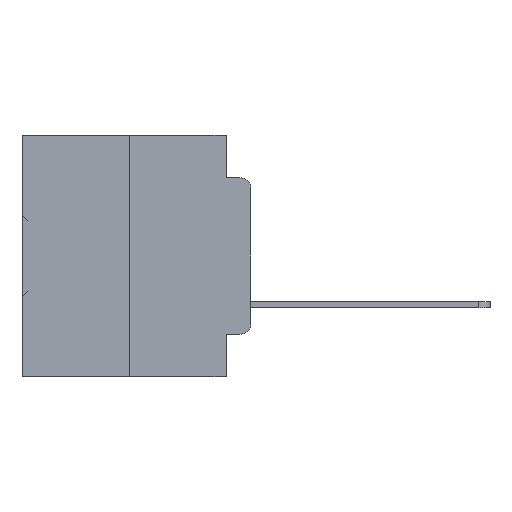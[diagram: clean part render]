
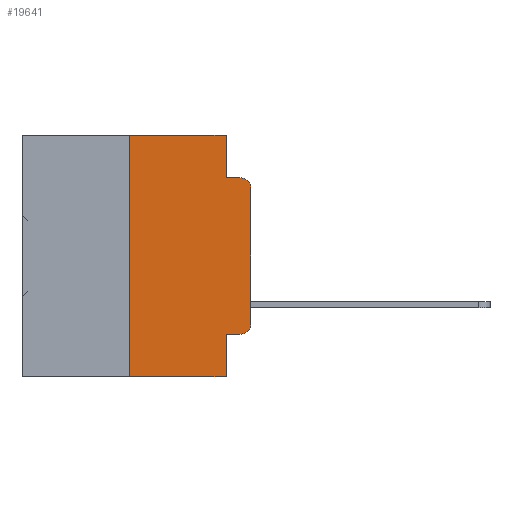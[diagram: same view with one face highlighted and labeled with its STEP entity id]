
A CAD part, left-side view. The second image highlights one B-rep face of the part: STEP entity #19641.
In plain terms, the highlighted planar face has unit normal (-1, 0, 0).
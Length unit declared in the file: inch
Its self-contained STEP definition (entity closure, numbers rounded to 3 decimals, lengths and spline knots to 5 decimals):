
#29 = CARTESIAN_POINT ( 'NONE',  ( 0., 0.25, 0. ) ) ;
#360 = DIRECTION ( 'NONE',  ( 0., -1., 0. ) ) ;
#1516 = VERTEX_POINT ( 'NONE', #3361 ) ;
#1761 = CIRCLE ( 'NONE', #10310, 0.02 ) ;
#1871 = PLANE ( 'NONE',  #21102 ) ;
#1958 = DIRECTION ( 'NONE',  ( 0., -1., 0. ) ) ;
#2050 = DIRECTION ( 'NONE',  ( 0., 0., -1. ) ) ;
#2464 = CARTESIAN_POINT ( 'NONE',  ( 0., 0.25, -0.5 ) ) ;
#2479 = CARTESIAN_POINT ( 'NONE',  ( 0., 0.051, 0. ) ) ;
#3361 = CARTESIAN_POINT ( 'NONE',  ( 0., 0.02, -0.4115 ) ) ;
#4525 = LINE ( 'NONE', #7889, #23903 ) ;
#4834 = DIRECTION ( 'NONE',  ( 1., 0., 0. ) ) ;
#5090 = DIRECTION ( 'NONE',  ( 0., 0., -1. ) ) ;
#5149 = CARTESIAN_POINT ( 'NONE',  ( 0., 0.02, -0.1085 ) ) ;
#5517 = EDGE_CURVE ( 'NONE', #33717, #28321, #29204, .T. ) ;
#5918 = ORIENTED_EDGE ( 'NONE', *, *, #34661, .F. ) ;
#6010 = CARTESIAN_POINT ( 'NONE',  ( 0., 0.25, 0. ) ) ;
#7038 = CARTESIAN_POINT ( 'NONE',  ( 0., 0., -0.1085 ) ) ;
#7889 = CARTESIAN_POINT ( 'NONE',  ( 0., 0.473, -0.5 ) ) ;
#9245 = ORIENTED_EDGE ( 'NONE', *, *, #11551, .T. ) ;
#9470 = DIRECTION ( 'NONE',  ( 0., 0., 1. ) ) ;
#10193 = VECTOR ( 'NONE', #360, 39.37008 ) ;
#10310 = AXIS2_PLACEMENT_3D ( 'NONE', #5149, #25488, #2050 ) ;
#10795 = DIRECTION ( 'NONE',  ( 0., -1., 0. ) ) ;
#11041 = CARTESIAN_POINT ( 'NONE',  ( 0., 0.051, -0.4115 ) ) ;
#11551 = EDGE_CURVE ( 'NONE', #26142, #1516, #20433, .T. ) ;
#13158 = EDGE_CURVE ( 'NONE', #28321, #17283, #20292, .T. ) ;
#13922 = VECTOR ( 'NONE', #1958, 39.37008 ) ;
#14034 = ORIENTED_EDGE ( 'NONE', *, *, #37414, .T. ) ;
#15001 = ORIENTED_EDGE ( 'NONE', *, *, #5517, .F. ) ;
#15716 = LINE ( 'NONE', #24200, #10193 ) ;
#16428 = CARTESIAN_POINT ( 'NONE',  ( 0., 0.02, -0.0885 ) ) ;
#16516 = CARTESIAN_POINT ( 'NONE',  ( 0., 0.473, 0. ) ) ;
#16660 = CARTESIAN_POINT ( 'NONE',  ( 0., 0., 0. ) ) ;
#16701 = CARTESIAN_POINT ( 'NONE',  ( 0., 0.051, 0. ) ) ;
#17232 = DIRECTION ( 'NONE',  ( 0., 0., -1. ) ) ;
#17283 = VERTEX_POINT ( 'NONE', #16701 ) ;
#17725 = CARTESIAN_POINT ( 'NONE',  ( 0., 0.02, -0.3915 ) ) ;
#19314 = VECTOR ( 'NONE', #19717, 39.37008 ) ;
#19569 = ORIENTED_EDGE ( 'NONE', *, *, #36699, .T. ) ;
#19637 = VERTEX_POINT ( 'NONE', #16428 ) ;
#19641 = ADVANCED_FACE ( 'NONE', ( #25426 ), #1871, .F. ) ;
#19717 = DIRECTION ( 'NONE',  ( 0., 0., 1. ) ) ;
#20061 = VERTEX_POINT ( 'NONE', #31621 ) ;
#20292 = LINE ( 'NONE', #16516, #13922 ) ;
#20334 = EDGE_CURVE ( 'NONE', #30525, #19637, #15716, .T. ) ;
#20433 = LINE ( 'NONE', #11041, #37977 ) ;
#20505 = VECTOR ( 'NONE', #5090, 39.37008 ) ;
#21102 = AXIS2_PLACEMENT_3D ( 'NONE', #31077, #4834, #25412 ) ;
#21633 = ORIENTED_EDGE ( 'NONE', *, *, #35663, .T. ) ;
#21727 = CIRCLE ( 'NONE', #21842, 0.02 ) ;
#21842 = AXIS2_PLACEMENT_3D ( 'NONE', #17725, #26381, #17232 ) ;
#22812 = LINE ( 'NONE', #35912, #30615 ) ;
#23273 = EDGE_CURVE ( 'NONE', #26142, #20061, #31541, .T. ) ;
#23319 = ORIENTED_EDGE ( 'NONE', *, *, #20334, .F. ) ;
#23903 = VECTOR ( 'NONE', #31759, 39.37008 ) ;
#24200 = CARTESIAN_POINT ( 'NONE',  ( 0., 0.051, -0.0885 ) ) ;
#24656 = ORIENTED_EDGE ( 'NONE', *, *, #13158, .F. ) ;
#24825 = VERTEX_POINT ( 'NONE', #32892 ) ;
#25412 = DIRECTION ( 'NONE',  ( 0., 0., -1. ) ) ;
#25426 = FACE_OUTER_BOUND ( 'NONE', #35416, .T. ) ;
#25488 = DIRECTION ( 'NONE',  ( -1., 0., 0. ) ) ;
#26142 = VERTEX_POINT ( 'NONE', #33833 ) ;
#26381 = DIRECTION ( 'NONE',  ( -1., 0., 0. ) ) ;
#28321 = VERTEX_POINT ( 'NONE', #6010 ) ;
#29204 = LINE ( 'NONE', #29, #30583 ) ;
#30525 = VERTEX_POINT ( 'NONE', #36915 ) ;
#30583 = VECTOR ( 'NONE', #9470, 39.37008 ) ;
#30615 = VECTOR ( 'NONE', #33944, 39.37008 ) ;
#30914 = VERTEX_POINT ( 'NONE', #7038 ) ;
#31077 = CARTESIAN_POINT ( 'NONE',  ( 0., 0.473, 0. ) ) ;
#31541 = LINE ( 'NONE', #2479, #20505 ) ;
#31621 = CARTESIAN_POINT ( 'NONE',  ( 0., 0.051, -0.5 ) ) ;
#31759 = DIRECTION ( 'NONE',  ( 0., -1., 0. ) ) ;
#32892 = CARTESIAN_POINT ( 'NONE',  ( 0., 0., -0.3915 ) ) ;
#33717 = VERTEX_POINT ( 'NONE', #2464 ) ;
#33833 = CARTESIAN_POINT ( 'NONE',  ( 0., 0.051, -0.4115 ) ) ;
#33944 = DIRECTION ( 'NONE',  ( 0., 0., -1. ) ) ;
#34661 = EDGE_CURVE ( 'NONE', #17283, #30525, #22812, .T. ) ;
#34966 = LINE ( 'NONE', #16660, #19314 ) ;
#35416 = EDGE_LOOP ( 'NONE', ( #19569, #36954, #23319, #5918, #24656, #15001, #14034, #35979, #9245, #21633 ) ) ;
#35663 = EDGE_CURVE ( 'NONE', #1516, #24825, #21727, .T. ) ;
#35912 = CARTESIAN_POINT ( 'NONE',  ( 0., 0.051, 0. ) ) ;
#35979 = ORIENTED_EDGE ( 'NONE', *, *, #23273, .F. ) ;
#36699 = EDGE_CURVE ( 'NONE', #24825, #30914, #34966, .T. ) ;
#36915 = CARTESIAN_POINT ( 'NONE',  ( 0., 0.051, -0.0885 ) ) ;
#36954 = ORIENTED_EDGE ( 'NONE', *, *, #37364, .T. ) ;
#37364 = EDGE_CURVE ( 'NONE', #30914, #19637, #1761, .T. ) ;
#37414 = EDGE_CURVE ( 'NONE', #33717, #20061, #4525, .T. ) ;
#37977 = VECTOR ( 'NONE', #10795, 39.37008 ) ;
